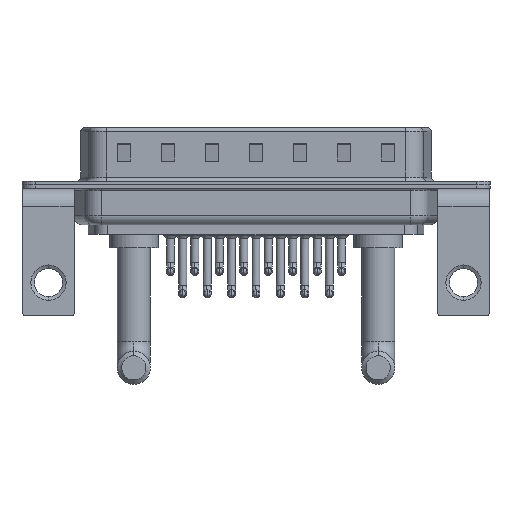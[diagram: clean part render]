
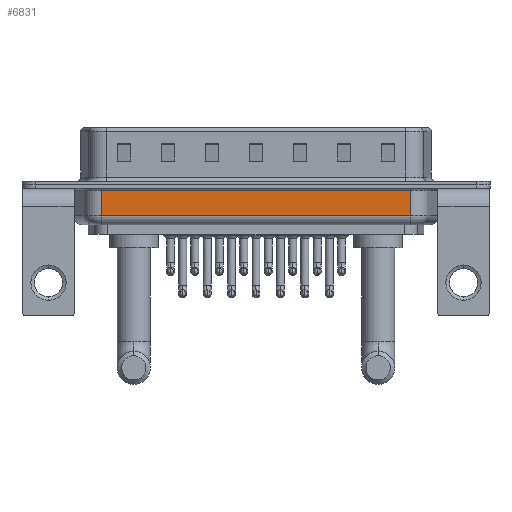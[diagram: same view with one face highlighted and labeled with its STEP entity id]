
A CAD part, front view. The second image highlights one B-rep face of the part: STEP entity #6831.
In plain terms, the highlighted planar face has unit normal (0, -1, 0).
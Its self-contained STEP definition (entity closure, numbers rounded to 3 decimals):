
#297 = VERTEX_POINT ( 'NONE', #13281 ) ;
#466 = EDGE_LOOP ( 'NONE', ( #1499, #20182, #21523, #24306 ) ) ;
#1347 = DIRECTION ( 'NONE',  ( 0., 1., 0. ) ) ;
#1499 = ORIENTED_EDGE ( 'NONE', *, *, #2756, .F. ) ;
#1503 = VECTOR ( 'NONE', #15094, 1000. ) ;
#1610 = FACE_OUTER_BOUND ( 'NONE', #466, .T. ) ;
#2756 = EDGE_CURVE ( 'NONE', #6908, #297, #3596, .T. ) ;
#3596 = LINE ( 'NONE', #21018, #1503 ) ;
#4091 = CARTESIAN_POINT ( 'NONE',  ( 41.044, -5.35, -3.5 ) ) ;
#4715 = VERTEX_POINT ( 'NONE', #4091 ) ;
#5463 = DIRECTION ( 'NONE',  ( -1., 0., 0. ) ) ;
#5588 = LINE ( 'NONE', #11152, #10497 ) ;
#6113 = DIRECTION ( 'NONE',  ( 0., 0., 1. ) ) ;
#6831 = ADVANCED_FACE ( 'NONE', ( #1610 ), #15173, .F. ) ;
#6908 = VERTEX_POINT ( 'NONE', #9098 ) ;
#6980 = EDGE_CURVE ( 'NONE', #4715, #12990, #25330, .T. ) ;
#8213 = CARTESIAN_POINT ( 'NONE',  ( 6.006, -5.35, -3.5 ) ) ;
#9098 = CARTESIAN_POINT ( 'NONE',  ( 6.006, -5.35, -3.5 ) ) ;
#10167 = VECTOR ( 'NONE', #23696, 1000. ) ;
#10497 = VECTOR ( 'NONE', #5463, 1000. ) ;
#11152 = CARTESIAN_POINT ( 'NONE',  ( 6.006, -5.35, -0.65 ) ) ;
#12990 = VERTEX_POINT ( 'NONE', #13380 ) ;
#13281 = CARTESIAN_POINT ( 'NONE',  ( 6.006, -5.35, -0.65 ) ) ;
#13380 = CARTESIAN_POINT ( 'NONE',  ( 41.044, -5.35, -0.65 ) ) ;
#13495 = EDGE_CURVE ( 'NONE', #12990, #297, #5588, .T. ) ;
#15094 = DIRECTION ( 'NONE',  ( 0., 0., 1. ) ) ;
#15173 = PLANE ( 'NONE',  #18174 ) ;
#18174 = AXIS2_PLACEMENT_3D ( 'NONE', #21090, #1347, #23040 ) ;
#20182 = ORIENTED_EDGE ( 'NONE', *, *, #25126, .T. ) ;
#21018 = CARTESIAN_POINT ( 'NONE',  ( 6.006, -5.35, -4.5 ) ) ;
#21090 = CARTESIAN_POINT ( 'NONE',  ( 6.006, -5.35, -4.5 ) ) ;
#21523 = ORIENTED_EDGE ( 'NONE', *, *, #6980, .T. ) ;
#22697 = VECTOR ( 'NONE', #6113, 1000. ) ;
#23040 = DIRECTION ( 'NONE',  ( 0., 0., 1. ) ) ;
#23661 = CARTESIAN_POINT ( 'NONE',  ( 41.044, -5.35, -4.5 ) ) ;
#23696 = DIRECTION ( 'NONE',  ( 1., 0., 0. ) ) ;
#24065 = LINE ( 'NONE', #8213, #10167 ) ;
#24306 = ORIENTED_EDGE ( 'NONE', *, *, #13495, .T. ) ;
#25126 = EDGE_CURVE ( 'NONE', #6908, #4715, #24065, .T. ) ;
#25330 = LINE ( 'NONE', #23661, #22697 ) ;
